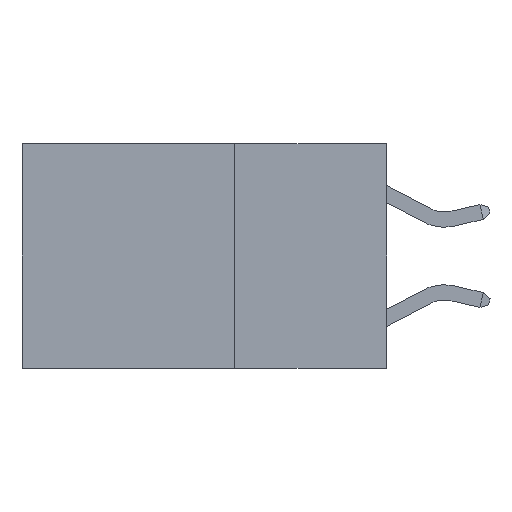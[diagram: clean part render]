
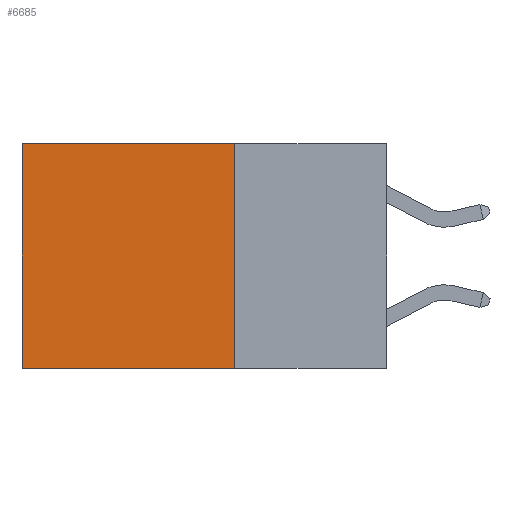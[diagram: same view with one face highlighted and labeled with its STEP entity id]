
A CAD part, left-side view. The second image highlights one B-rep face of the part: STEP entity #6685.
In plain terms, the highlighted planar face has unit normal (-1, 0, 0).
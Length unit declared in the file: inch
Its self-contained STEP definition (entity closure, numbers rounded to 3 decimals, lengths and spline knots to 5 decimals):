
#35 = CARTESIAN_POINT ( 'NONE',  ( 0.2625, 0.6, 0. ) ) ;
#302 = EDGE_CURVE ( 'NONE', #1719, #11631, #26920, .T. ) ;
#676 = DIRECTION ( 'NONE',  ( 0., 1., 0. ) ) ;
#1719 = VERTEX_POINT ( 'NONE', #16575 ) ;
#2405 = DIRECTION ( 'NONE',  ( 0., 0., -1. ) ) ;
#2696 = VERTEX_POINT ( 'NONE', #23060 ) ;
#2742 = FACE_OUTER_BOUND ( 'NONE', #6654, .T. ) ;
#3113 = ORIENTED_EDGE ( 'NONE', *, *, #302, .T. ) ;
#4287 = LINE ( 'NONE', #35, #19588 ) ;
#6654 = EDGE_LOOP ( 'NONE', ( #17863, #23506, #13513, #3113 ) ) ;
#6685 = ADVANCED_FACE ( 'NONE', ( #2742 ), #21081, .F. ) ;
#8304 = CARTESIAN_POINT ( 'NONE',  ( 0.2625, 0.25, 0. ) ) ;
#8992 = VECTOR ( 'NONE', #25167, 39.37008 ) ;
#9968 = VECTOR ( 'NONE', #676, 39.37008 ) ;
#10486 = DIRECTION ( 'NONE',  ( 1., 0., 0. ) ) ;
#10681 = VECTOR ( 'NONE', #25607, 39.37008 ) ;
#11631 = VERTEX_POINT ( 'NONE', #26223 ) ;
#12897 = CARTESIAN_POINT ( 'NONE',  ( 0.2625, 0.25, -0.37 ) ) ;
#13511 = VERTEX_POINT ( 'NONE', #18657 ) ;
#13513 = ORIENTED_EDGE ( 'NONE', *, *, #17357, .F. ) ;
#14825 = CARTESIAN_POINT ( 'NONE',  ( 0.2625, 0.25, 0. ) ) ;
#16575 = CARTESIAN_POINT ( 'NONE',  ( 0.2625, 0.25, 0. ) ) ;
#17357 = EDGE_CURVE ( 'NONE', #1719, #13511, #20334, .T. ) ;
#17563 = EDGE_CURVE ( 'NONE', #13511, #2696, #26942, .T. ) ;
#17863 = ORIENTED_EDGE ( 'NONE', *, *, #26530, .T. ) ;
#18657 = CARTESIAN_POINT ( 'NONE',  ( 0.2625, 0.25, -0.37 ) ) ;
#19588 = VECTOR ( 'NONE', #2405, 39.37008 ) ;
#20334 = LINE ( 'NONE', #23045, #8992 ) ;
#21081 = PLANE ( 'NONE',  #27512 ) ;
#23045 = CARTESIAN_POINT ( 'NONE',  ( 0.2625, 0.25, 0. ) ) ;
#23060 = CARTESIAN_POINT ( 'NONE',  ( 0.2625, 0.6, -0.37 ) ) ;
#23506 = ORIENTED_EDGE ( 'NONE', *, *, #17563, .F. ) ;
#25167 = DIRECTION ( 'NONE',  ( 0., 0., -1. ) ) ;
#25359 = DIRECTION ( 'NONE',  ( 0., 0., -1. ) ) ;
#25607 = DIRECTION ( 'NONE',  ( 0., 1., 0. ) ) ;
#26223 = CARTESIAN_POINT ( 'NONE',  ( 0.2625, 0.6, 0. ) ) ;
#26530 = EDGE_CURVE ( 'NONE', #11631, #2696, #4287, .T. ) ;
#26920 = LINE ( 'NONE', #14825, #9968 ) ;
#26942 = LINE ( 'NONE', #12897, #10681 ) ;
#27512 = AXIS2_PLACEMENT_3D ( 'NONE', #8304, #10486, #25359 ) ;
